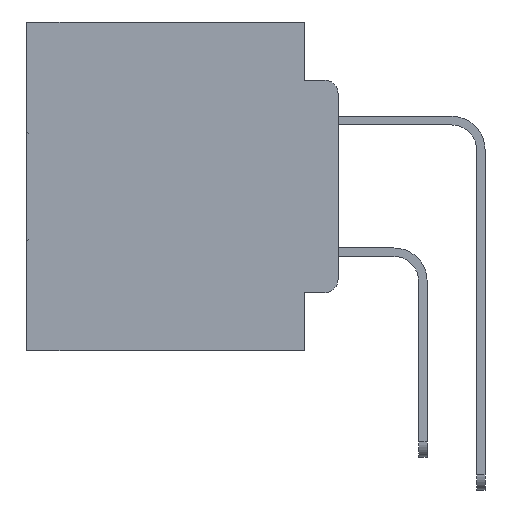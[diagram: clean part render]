
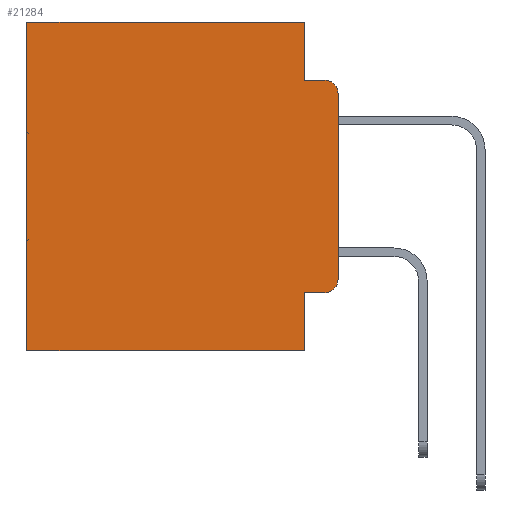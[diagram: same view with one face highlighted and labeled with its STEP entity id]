
A CAD part, left-side view. The second image highlights one B-rep face of the part: STEP entity #21284.
In plain terms, the highlighted planar face has unit normal (-1, 0, 0).
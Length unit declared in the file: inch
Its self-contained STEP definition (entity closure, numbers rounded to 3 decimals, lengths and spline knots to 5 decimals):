
#391 = ORIENTED_EDGE ( 'NONE', *, *, #19343, .T. ) ;
#1963 = DIRECTION ( 'NONE',  ( -1., 0., 0. ) ) ;
#2023 = VERTEX_POINT ( 'NONE', #28119 ) ;
#2730 = VECTOR ( 'NONE', #28882, 39.37008 ) ;
#2892 = VERTEX_POINT ( 'NONE', #14444 ) ;
#3681 = LINE ( 'NONE', #25674, #16823 ) ;
#3829 = VECTOR ( 'NONE', #18255, 39.37008 ) ;
#4217 = EDGE_CURVE ( 'NONE', #2892, #15854, #10842, .T. ) ;
#4704 = VECTOR ( 'NONE', #23444, 39.37008 ) ;
#5072 = EDGE_CURVE ( 'NONE', #9553, #2023, #17788, .T. ) ;
#6266 = ORIENTED_EDGE ( 'NONE', *, *, #11779, .F. ) ;
#6346 = CARTESIAN_POINT ( 'NONE',  ( 0.298, 0.051, 0. ) ) ;
#6605 = FACE_OUTER_BOUND ( 'NONE', #16704, .T. ) ;
#7047 = CARTESIAN_POINT ( 'NONE',  ( 0.298, 0.473, 0. ) ) ;
#7760 = CARTESIAN_POINT ( 'NONE',  ( 0.298, 0., 0. ) ) ;
#8038 = DIRECTION ( 'NONE',  ( 0., 0., -1. ) ) ;
#8913 = VERTEX_POINT ( 'NONE', #7047 ) ;
#9373 = DIRECTION ( 'NONE',  ( 0., 0., -1. ) ) ;
#9553 = VERTEX_POINT ( 'NONE', #14953 ) ;
#9568 = CARTESIAN_POINT ( 'NONE',  ( 0.298, 0.02, -0.1085 ) ) ;
#10221 = AXIS2_PLACEMENT_3D ( 'NONE', #9568, #27785, #12189 ) ;
#10271 = DIRECTION ( 'NONE',  ( 0., 0., -1. ) ) ;
#10309 = CARTESIAN_POINT ( 'NONE',  ( 0.298, 0., 0. ) ) ;
#10474 = VECTOR ( 'NONE', #29823, 39.37008 ) ;
#10790 = VECTOR ( 'NONE', #8038, 39.37008 ) ;
#10794 = LINE ( 'NONE', #10309, #3829 ) ;
#10842 = LINE ( 'NONE', #16211, #23110 ) ;
#11420 = EDGE_CURVE ( 'NONE', #18456, #2892, #24672, .T. ) ;
#11779 = EDGE_CURVE ( 'NONE', #31895, #26301, #27854, .T. ) ;
#12031 = ORIENTED_EDGE ( 'NONE', *, *, #23419, .F. ) ;
#12189 = DIRECTION ( 'NONE',  ( 0., 0., -1. ) ) ;
#13491 = ORIENTED_EDGE ( 'NONE', *, *, #11420, .F. ) ;
#13720 = ORIENTED_EDGE ( 'NONE', *, *, #4217, .F. ) ;
#13973 = DIRECTION ( 'NONE',  ( 1., 0., 0. ) ) ;
#14444 = CARTESIAN_POINT ( 'NONE',  ( 0.298, 0.051, -0.5 ) ) ;
#14889 = VECTOR ( 'NONE', #9373, 39.37008 ) ;
#14953 = CARTESIAN_POINT ( 'NONE',  ( 0.298, 0.02, -0.4115 ) ) ;
#15103 = ORIENTED_EDGE ( 'NONE', *, *, #33478, .T. ) ;
#15234 = VERTEX_POINT ( 'NONE', #28753 ) ;
#15854 = VERTEX_POINT ( 'NONE', #25149 ) ;
#16211 = CARTESIAN_POINT ( 'NONE',  ( 0.298, 0., -0.5 ) ) ;
#16672 = ORIENTED_EDGE ( 'NONE', *, *, #30242, .T. ) ;
#16704 = EDGE_LOOP ( 'NONE', ( #26405, #16672, #12031, #6266, #391, #15103, #13720, #13491, #24306, #18050 ) ) ;
#16823 = VECTOR ( 'NONE', #10271, 39.37008 ) ;
#17648 = CARTESIAN_POINT ( 'NONE',  ( 0.298, 0.02, -0.3915 ) ) ;
#17788 = CIRCLE ( 'NONE', #31633, 0.02 ) ;
#18050 = ORIENTED_EDGE ( 'NONE', *, *, #5072, .T. ) ;
#18255 = DIRECTION ( 'NONE',  ( 0., 0., -1. ) ) ;
#18456 = VERTEX_POINT ( 'NONE', #32531 ) ;
#19343 = EDGE_CURVE ( 'NONE', #31895, #8913, #31508, .T. ) ;
#20237 = DIRECTION ( 'NONE',  ( 0., 0., -1. ) ) ;
#20661 = CIRCLE ( 'NONE', #10221, 0.02 ) ;
#20771 = VERTEX_POINT ( 'NONE', #32468 ) ;
#21224 = CARTESIAN_POINT ( 'NONE',  ( 0.298, 0.051, -0.0885 ) ) ;
#21284 = ADVANCED_FACE ( 'NONE', ( #6605 ), #29454, .F. ) ;
#21712 = CARTESIAN_POINT ( 'NONE',  ( 0.298, 0., 0. ) ) ;
#23110 = VECTOR ( 'NONE', #26527, 39.37008 ) ;
#23419 = EDGE_CURVE ( 'NONE', #26301, #15234, #30326, .T. ) ;
#23444 = DIRECTION ( 'NONE',  ( 0., 1., 0. ) ) ;
#24306 = ORIENTED_EDGE ( 'NONE', *, *, #29464, .T. ) ;
#24492 = EDGE_CURVE ( 'NONE', #20771, #2023, #10794, .T. ) ;
#24672 = LINE ( 'NONE', #31269, #10790 ) ;
#25014 = CARTESIAN_POINT ( 'NONE',  ( 0.298, 0.051, 0. ) ) ;
#25149 = CARTESIAN_POINT ( 'NONE',  ( 0.298, 0.473, -0.5 ) ) ;
#25158 = LINE ( 'NONE', #27289, #10474 ) ;
#25674 = CARTESIAN_POINT ( 'NONE',  ( 0.298, 0.473, 0. ) ) ;
#26301 = VERTEX_POINT ( 'NONE', #32510 ) ;
#26405 = ORIENTED_EDGE ( 'NONE', *, *, #24492, .F. ) ;
#26527 = DIRECTION ( 'NONE',  ( 0., 1., 0. ) ) ;
#27289 = CARTESIAN_POINT ( 'NONE',  ( 0.298, 0.051, -0.4115 ) ) ;
#27785 = DIRECTION ( 'NONE',  ( -1., 0., 0. ) ) ;
#27854 = LINE ( 'NONE', #25014, #14889 ) ;
#28119 = CARTESIAN_POINT ( 'NONE',  ( 0.298, 0., -0.3915 ) ) ;
#28753 = CARTESIAN_POINT ( 'NONE',  ( 0.298, 0.02, -0.0885 ) ) ;
#28882 = DIRECTION ( 'NONE',  ( 0., -1., 0. ) ) ;
#29454 = PLANE ( 'NONE',  #31299 ) ;
#29464 = EDGE_CURVE ( 'NONE', #18456, #9553, #25158, .T. ) ;
#29823 = DIRECTION ( 'NONE',  ( 0., -1., 0. ) ) ;
#30242 = EDGE_CURVE ( 'NONE', #20771, #15234, #20661, .T. ) ;
#30326 = LINE ( 'NONE', #21224, #2730 ) ;
#31269 = CARTESIAN_POINT ( 'NONE',  ( 0.298, 0.051, 0. ) ) ;
#31299 = AXIS2_PLACEMENT_3D ( 'NONE', #21712, #13973, #31987 ) ;
#31508 = LINE ( 'NONE', #7760, #4704 ) ;
#31633 = AXIS2_PLACEMENT_3D ( 'NONE', #17648, #1963, #20237 ) ;
#31895 = VERTEX_POINT ( 'NONE', #6346 ) ;
#31987 = DIRECTION ( 'NONE',  ( 0., 0., -1. ) ) ;
#32468 = CARTESIAN_POINT ( 'NONE',  ( 0.298, 0., -0.1085 ) ) ;
#32510 = CARTESIAN_POINT ( 'NONE',  ( 0.298, 0.051, -0.0885 ) ) ;
#32531 = CARTESIAN_POINT ( 'NONE',  ( 0.298, 0.051, -0.4115 ) ) ;
#33478 = EDGE_CURVE ( 'NONE', #8913, #15854, #3681, .T. ) ;
